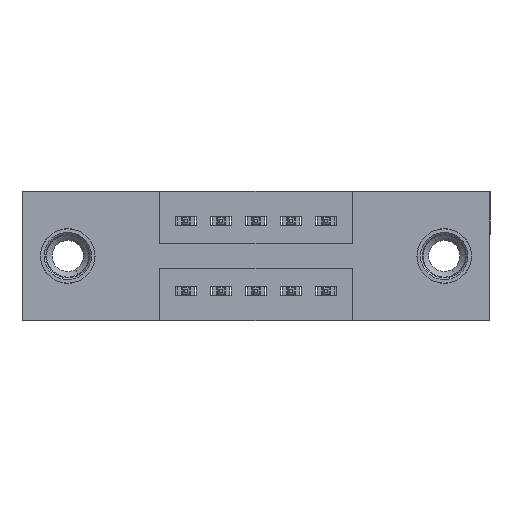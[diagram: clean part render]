
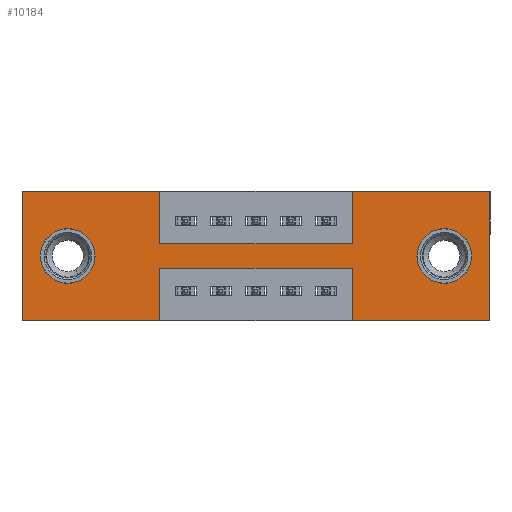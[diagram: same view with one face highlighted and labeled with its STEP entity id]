
A CAD part, front view. The second image highlights one B-rep face of the part: STEP entity #10184.
In plain terms, the highlighted planar face has unit normal (0, -1, 0).
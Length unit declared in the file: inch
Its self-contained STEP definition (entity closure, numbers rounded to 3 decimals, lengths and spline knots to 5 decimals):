
#84 = ORIENTED_EDGE ( 'NONE', *, *, #1276, .F. ) ;
#183 = VERTEX_POINT ( 'NONE', #9465 ) ;
#184 = LINE ( 'NONE', #3581, #257 ) ;
#246 = CIRCLE ( 'NONE', #9454, 0.078 ) ;
#257 = VECTOR ( 'NONE', #7039, 39.37008 ) ;
#346 = VERTEX_POINT ( 'NONE', #5583 ) ;
#485 = CARTESIAN_POINT ( 'NONE',  ( 0.3925, 0., 0. ) ) ;
#497 = DIRECTION ( 'NONE',  ( 0., 1., 0. ) ) ;
#583 = EDGE_CURVE ( 'NONE', #183, #6544, #6311, .T. ) ;
#666 = VERTEX_POINT ( 'NONE', #3781 ) ;
#695 = ORIENTED_EDGE ( 'NONE', *, *, #4826, .F. ) ;
#701 = EDGE_CURVE ( 'NONE', #10505, #666, #4126, .T. ) ;
#827 = CARTESIAN_POINT ( 'NONE',  ( 0.13, 0., -0.185 ) ) ;
#893 = CARTESIAN_POINT ( 'NONE',  ( 0., 0., 0. ) ) ;
#1205 = EDGE_CURVE ( 'NONE', #2777, #3181, #3511, .T. ) ;
#1233 = DIRECTION ( 'NONE',  ( 0., 0., 1. ) ) ;
#1276 = EDGE_CURVE ( 'NONE', #6830, #10505, #8635, .T. ) ;
#1555 = DIRECTION ( 'NONE',  ( 0., 0., -1. ) ) ;
#1628 = CARTESIAN_POINT ( 'NONE',  ( 1.205, 0., -0.185 ) ) ;
#1630 = VERTEX_POINT ( 'NONE', #2434 ) ;
#1632 = ORIENTED_EDGE ( 'NONE', *, *, #10116, .F. ) ;
#1677 = DIRECTION ( 'NONE',  ( -1., 0., 0. ) ) ;
#1820 = DIRECTION ( 'NONE',  ( 1., 0., 0. ) ) ;
#1918 = EDGE_LOOP ( 'NONE', ( #4781, #7637 ) ) ;
#1977 = CARTESIAN_POINT ( 'NONE',  ( 0.13, 0., -0.263 ) ) ;
#2291 = CARTESIAN_POINT ( 'NONE',  ( 0.13, 0., -0.185 ) ) ;
#2362 = EDGE_CURVE ( 'NONE', #1630, #3121, #10347, .T. ) ;
#2376 = DIRECTION ( 'NONE',  ( 0., 0., -1. ) ) ;
#2434 = CARTESIAN_POINT ( 'NONE',  ( 0.13, 0., -0.107 ) ) ;
#2490 = ORIENTED_EDGE ( 'NONE', *, *, #5869, .T. ) ;
#2544 = CARTESIAN_POINT ( 'NONE',  ( 0.3925, 0., -0.15 ) ) ;
#2555 = DIRECTION ( 'NONE',  ( 0., 1., 0. ) ) ;
#2601 = EDGE_CURVE ( 'NONE', #9821, #9460, #5728, .T. ) ;
#2644 = VERTEX_POINT ( 'NONE', #7766 ) ;
#2745 = EDGE_CURVE ( 'NONE', #2644, #10741, #246, .T. ) ;
#2764 = ORIENTED_EDGE ( 'NONE', *, *, #4087, .F. ) ;
#2765 = VECTOR ( 'NONE', #6841, 39.37008 ) ;
#2777 = VERTEX_POINT ( 'NONE', #9427 ) ;
#2936 = CARTESIAN_POINT ( 'NONE',  ( 0., 0., -0.37 ) ) ;
#2981 = ORIENTED_EDGE ( 'NONE', *, *, #4518, .F. ) ;
#3021 = ORIENTED_EDGE ( 'NONE', *, *, #4507, .F. ) ;
#3121 = VERTEX_POINT ( 'NONE', #1977 ) ;
#3181 = VERTEX_POINT ( 'NONE', #10188 ) ;
#3211 = LINE ( 'NONE', #4853, #6920 ) ;
#3230 = LINE ( 'NONE', #7765, #9531 ) ;
#3394 = DIRECTION ( 'NONE',  ( 0., -1., 0. ) ) ;
#3511 = LINE ( 'NONE', #5266, #3611 ) ;
#3581 = CARTESIAN_POINT ( 'NONE',  ( 0.9425, 0., -0.37 ) ) ;
#3611 = VECTOR ( 'NONE', #1233, 39.37008 ) ;
#3781 = CARTESIAN_POINT ( 'NONE',  ( 0.3925, 0., -0.15 ) ) ;
#3860 = AXIS2_PLACEMENT_3D ( 'NONE', #8030, #8954, #4622 ) ;
#4074 = CARTESIAN_POINT ( 'NONE',  ( 0., 0., 0. ) ) ;
#4087 = EDGE_CURVE ( 'NONE', #666, #2777, #9474, .T. ) ;
#4125 = ORIENTED_EDGE ( 'NONE', *, *, #5514, .F. ) ;
#4126 = LINE ( 'NONE', #8319, #9782 ) ;
#4192 = DIRECTION ( 'NONE',  ( 0., 0., 1. ) ) ;
#4197 = FACE_BOUND ( 'NONE', #10637, .T. ) ;
#4370 = VECTOR ( 'NONE', #9781, 39.37008 ) ;
#4507 = EDGE_CURVE ( 'NONE', #346, #183, #184, .T. ) ;
#4518 = EDGE_CURVE ( 'NONE', #10876, #10536, #10838, .T. ) ;
#4622 = DIRECTION ( 'NONE',  ( 0., 0., -1. ) ) ;
#4781 = ORIENTED_EDGE ( 'NONE', *, *, #2362, .T. ) ;
#4826 = EDGE_CURVE ( 'NONE', #9460, #6830, #9435, .T. ) ;
#4853 = CARTESIAN_POINT ( 'NONE',  ( 0.3925, 0., -0.37 ) ) ;
#4922 = CARTESIAN_POINT ( 'NONE',  ( 1.335, 0., -0.37 ) ) ;
#4967 = ORIENTED_EDGE ( 'NONE', *, *, #2745, .T. ) ;
#5042 = DIRECTION ( 'NONE',  ( 0., 0., -1. ) ) ;
#5100 = FACE_BOUND ( 'NONE', #1918, .T. ) ;
#5266 = CARTESIAN_POINT ( 'NONE',  ( 0.9425, 0., 0. ) ) ;
#5514 = EDGE_CURVE ( 'NONE', #6544, #9821, #3211, .T. ) ;
#5568 = ORIENTED_EDGE ( 'NONE', *, *, #1205, .F. ) ;
#5583 = CARTESIAN_POINT ( 'NONE',  ( 0.9425, 0., -0.37 ) ) ;
#5728 = LINE ( 'NONE', #10163, #6858 ) ;
#5844 = CIRCLE ( 'NONE', #3860, 0.078 ) ;
#5869 = EDGE_CURVE ( 'NONE', #10741, #2644, #5844, .T. ) ;
#5891 = DIRECTION ( 'NONE',  ( 0., 1., 0. ) ) ;
#6305 = ORIENTED_EDGE ( 'NONE', *, *, #8874, .F. ) ;
#6311 = LINE ( 'NONE', #8798, #9059 ) ;
#6419 = CARTESIAN_POINT ( 'NONE',  ( 1.335, 0., 0. ) ) ;
#6521 = VECTOR ( 'NONE', #1820, 39.37008 ) ;
#6544 = VERTEX_POINT ( 'NONE', #8678 ) ;
#6777 = AXIS2_PLACEMENT_3D ( 'NONE', #8572, #3394, #6844 ) ;
#6830 = VERTEX_POINT ( 'NONE', #4074 ) ;
#6841 = DIRECTION ( 'NONE',  ( -1., 0., 0. ) ) ;
#6844 = DIRECTION ( 'NONE',  ( 0., 0., -1. ) ) ;
#6858 = VECTOR ( 'NONE', #1677, 39.37008 ) ;
#6920 = VECTOR ( 'NONE', #1555, 39.37008 ) ;
#6971 = CARTESIAN_POINT ( 'NONE',  ( 0., 0., 0. ) ) ;
#7014 = DIRECTION ( 'NONE',  ( -1., 0., 0. ) ) ;
#7039 = DIRECTION ( 'NONE',  ( 0., 0., 1. ) ) ;
#7315 = DIRECTION ( 'NONE',  ( 0., 0., 1. ) ) ;
#7637 = ORIENTED_EDGE ( 'NONE', *, *, #10052, .T. ) ;
#7651 = FACE_OUTER_BOUND ( 'NONE', #10167, .T. ) ;
#7708 = LINE ( 'NONE', #2936, #2765 ) ;
#7765 = CARTESIAN_POINT ( 'NONE',  ( 0., 0., 0. ) ) ;
#7766 = CARTESIAN_POINT ( 'NONE',  ( 1.205, 0., -0.107 ) ) ;
#8030 = CARTESIAN_POINT ( 'NONE',  ( 1.205, 0., -0.185 ) ) ;
#8143 = CARTESIAN_POINT ( 'NONE',  ( 1.335, 0., 0. ) ) ;
#8167 = AXIS2_PLACEMENT_3D ( 'NONE', #827, #5891, #4192 ) ;
#8319 = CARTESIAN_POINT ( 'NONE',  ( 0.3925, 0., 0. ) ) ;
#8467 = DIRECTION ( 'NONE',  ( 1., 0., 0. ) ) ;
#8572 = CARTESIAN_POINT ( 'NONE',  ( 0., 0., -0.37 ) ) ;
#8635 = LINE ( 'NONE', #893, #10501 ) ;
#8678 = CARTESIAN_POINT ( 'NONE',  ( 0.3925, 0., -0.22 ) ) ;
#8798 = CARTESIAN_POINT ( 'NONE',  ( 0.3925, 0., -0.22 ) ) ;
#8874 = EDGE_CURVE ( 'NONE', #10536, #346, #7708, .T. ) ;
#8954 = DIRECTION ( 'NONE',  ( 0., 1., 0. ) ) ;
#9059 = VECTOR ( 'NONE', #7014, 39.37008 ) ;
#9155 = CIRCLE ( 'NONE', #10611, 0.078 ) ;
#9386 = CARTESIAN_POINT ( 'NONE',  ( 0.3925, 0., -0.37 ) ) ;
#9427 = CARTESIAN_POINT ( 'NONE',  ( 0.9425, 0., -0.15 ) ) ;
#9435 = LINE ( 'NONE', #6971, #9828 ) ;
#9454 = AXIS2_PLACEMENT_3D ( 'NONE', #1628, #2555, #5042 ) ;
#9460 = VERTEX_POINT ( 'NONE', #9748 ) ;
#9465 = CARTESIAN_POINT ( 'NONE',  ( 0.9425, 0., -0.22 ) ) ;
#9474 = LINE ( 'NONE', #2544, #6521 ) ;
#9531 = VECTOR ( 'NONE', #8467, 39.37008 ) ;
#9543 = DIRECTION ( 'NONE',  ( 0., 0., 1. ) ) ;
#9608 = ORIENTED_EDGE ( 'NONE', *, *, #2601, .F. ) ;
#9748 = CARTESIAN_POINT ( 'NONE',  ( 0., 0., -0.37 ) ) ;
#9781 = DIRECTION ( 'NONE',  ( 0., 0., -1. ) ) ;
#9782 = VECTOR ( 'NONE', #2376, 39.37008 ) ;
#9821 = VERTEX_POINT ( 'NONE', #9386 ) ;
#9828 = VECTOR ( 'NONE', #9543, 39.37008 ) ;
#10052 = EDGE_CURVE ( 'NONE', #3121, #1630, #9155, .T. ) ;
#10116 = EDGE_CURVE ( 'NONE', #3181, #10876, #3230, .T. ) ;
#10163 = CARTESIAN_POINT ( 'NONE',  ( 0., 0., -0.37 ) ) ;
#10167 = EDGE_LOOP ( 'NONE', ( #4125, #10847, #3021, #6305, #2981, #1632, #5568, #2764, #10455, #84, #695, #9608 ) ) ;
#10184 = ADVANCED_FACE ( 'NONE', ( #4197, #5100, #7651 ), #11120, .T. ) ;
#10188 = CARTESIAN_POINT ( 'NONE',  ( 0.9425, 0., 0. ) ) ;
#10347 = CIRCLE ( 'NONE', #8167, 0.078 ) ;
#10394 = DIRECTION ( 'NONE',  ( 1., 0., 0. ) ) ;
#10455 = ORIENTED_EDGE ( 'NONE', *, *, #701, .F. ) ;
#10501 = VECTOR ( 'NONE', #10394, 39.37008 ) ;
#10505 = VERTEX_POINT ( 'NONE', #485 ) ;
#10536 = VERTEX_POINT ( 'NONE', #4922 ) ;
#10538 = CARTESIAN_POINT ( 'NONE',  ( 1.205, 0., -0.263 ) ) ;
#10611 = AXIS2_PLACEMENT_3D ( 'NONE', #2291, #497, #7315 ) ;
#10637 = EDGE_LOOP ( 'NONE', ( #4967, #2490 ) ) ;
#10741 = VERTEX_POINT ( 'NONE', #10538 ) ;
#10838 = LINE ( 'NONE', #6419, #4370 ) ;
#10847 = ORIENTED_EDGE ( 'NONE', *, *, #583, .F. ) ;
#10876 = VERTEX_POINT ( 'NONE', #8143 ) ;
#11120 = PLANE ( 'NONE',  #6777 ) ;
